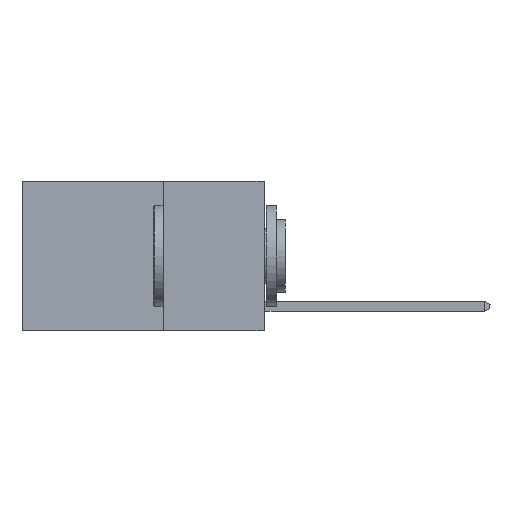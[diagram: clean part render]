
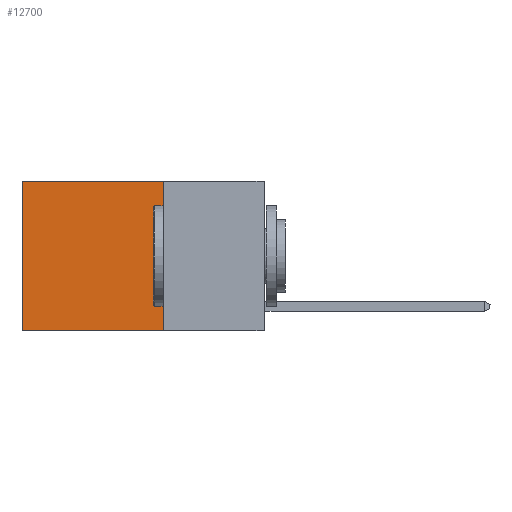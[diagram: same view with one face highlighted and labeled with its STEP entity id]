
A CAD part, left-side view. The second image highlights one B-rep face of the part: STEP entity #12700.
In plain terms, the highlighted planar face has unit normal (-1, 0, 0).
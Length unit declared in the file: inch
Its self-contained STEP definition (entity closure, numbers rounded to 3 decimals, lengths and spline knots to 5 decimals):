
#147 = LINE ( 'NONE', #4896, #5284 ) ;
#173 = VECTOR ( 'NONE', #15114, 39.37008 ) ;
#984 = VECTOR ( 'NONE', #10096, 39.37008 ) ;
#1039 = EDGE_CURVE ( 'NONE', #9475, #14355, #10327, .T. ) ;
#1275 = VERTEX_POINT ( 'NONE', #9680 ) ;
#2114 = EDGE_LOOP ( 'NONE', ( #6563, #6979, #7364, #9530 ) ) ;
#2504 = VERTEX_POINT ( 'NONE', #8193 ) ;
#2810 = DIRECTION ( 'NONE',  ( 0., 0., -1. ) ) ;
#3564 = CARTESIAN_POINT ( 'NONE',  ( 0.2625, 0.25, -0.37 ) ) ;
#3733 = FACE_OUTER_BOUND ( 'NONE', #2114, .T. ) ;
#3888 = VECTOR ( 'NONE', #2810, 39.37008 ) ;
#3983 = LINE ( 'NONE', #13574, #3888 ) ;
#4896 = CARTESIAN_POINT ( 'NONE',  ( 0.2625, 0.25, -0.37 ) ) ;
#5284 = VECTOR ( 'NONE', #9705, 39.37008 ) ;
#6563 = ORIENTED_EDGE ( 'NONE', *, *, #15224, .T. ) ;
#6584 = EDGE_CURVE ( 'NONE', #9475, #1275, #14638, .T. ) ;
#6979 = ORIENTED_EDGE ( 'NONE', *, *, #11140, .F. ) ;
#7117 = CARTESIAN_POINT ( 'NONE',  ( 0.2625, 0.25, 0. ) ) ;
#7364 = ORIENTED_EDGE ( 'NONE', *, *, #1039, .F. ) ;
#7955 = CARTESIAN_POINT ( 'NONE',  ( 0.2625, 0.25, 0. ) ) ;
#8193 = CARTESIAN_POINT ( 'NONE',  ( 0.2625, 0.6, -0.37 ) ) ;
#9475 = VERTEX_POINT ( 'NONE', #14212 ) ;
#9530 = ORIENTED_EDGE ( 'NONE', *, *, #6584, .T. ) ;
#9680 = CARTESIAN_POINT ( 'NONE',  ( 0.2625, 0.6, 0. ) ) ;
#9705 = DIRECTION ( 'NONE',  ( 0., 1., 0. ) ) ;
#9709 = DIRECTION ( 'NONE',  ( 0., 0., -1. ) ) ;
#10096 = DIRECTION ( 'NONE',  ( 0., 1., 0. ) ) ;
#10327 = LINE ( 'NONE', #7955, #173 ) ;
#10822 = PLANE ( 'NONE',  #14358 ) ;
#11140 = EDGE_CURVE ( 'NONE', #14355, #2504, #147, .T. ) ;
#11193 = CARTESIAN_POINT ( 'NONE',  ( 0.2625, 0.25, 0. ) ) ;
#11920 = DIRECTION ( 'NONE',  ( 1., 0., 0. ) ) ;
#12700 = ADVANCED_FACE ( 'NONE', ( #3733 ), #10822, .F. ) ;
#13574 = CARTESIAN_POINT ( 'NONE',  ( 0.2625, 0.6, 0. ) ) ;
#14212 = CARTESIAN_POINT ( 'NONE',  ( 0.2625, 0.25, 0. ) ) ;
#14355 = VERTEX_POINT ( 'NONE', #3564 ) ;
#14358 = AXIS2_PLACEMENT_3D ( 'NONE', #7117, #11920, #9709 ) ;
#14638 = LINE ( 'NONE', #11193, #984 ) ;
#15114 = DIRECTION ( 'NONE',  ( 0., 0., -1. ) ) ;
#15224 = EDGE_CURVE ( 'NONE', #1275, #2504, #3983, .T. ) ;
